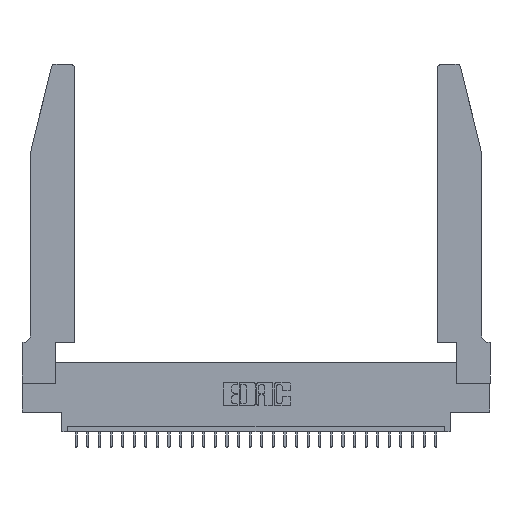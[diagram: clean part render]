
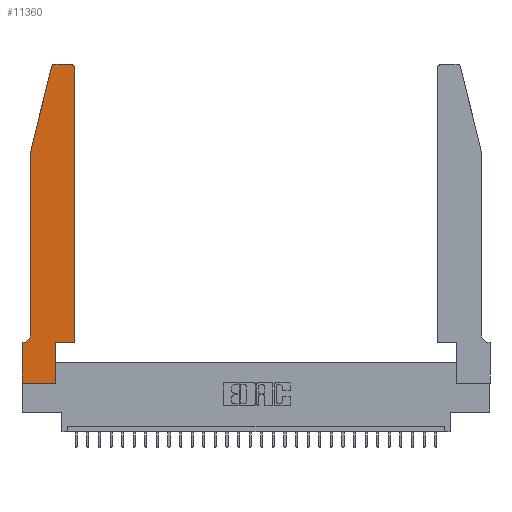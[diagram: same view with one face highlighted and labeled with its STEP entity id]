
A CAD part, top view. The second image highlights one B-rep face of the part: STEP entity #11360.
In plain terms, the highlighted planar face has unit normal (0, 0, 1).
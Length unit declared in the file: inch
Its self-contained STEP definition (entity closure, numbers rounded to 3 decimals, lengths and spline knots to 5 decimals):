
#20 = CARTESIAN_POINT ( 'NONE',  ( 0.4505, 0.35, 0.37 ) ) ;
#382 = VERTEX_POINT ( 'NONE', #9187 ) ;
#573 = CARTESIAN_POINT ( 'NONE',  ( 0.2865, 0.35, 0.37 ) ) ;
#619 = CARTESIAN_POINT ( 'NONE',  ( 0.0755, 0.35, 0.37 ) ) ;
#842 = DIRECTION ( 'NONE',  ( -1., 0., 0. ) ) ;
#876 = ORIENTED_EDGE ( 'NONE', *, *, #18215, .T. ) ;
#1455 = DIRECTION ( 'NONE',  ( 0., -1., 0. ) ) ;
#1483 = VERTEX_POINT ( 'NONE', #17665 ) ;
#1603 = CARTESIAN_POINT ( 'NONE',  ( 0., 0., 0.37 ) ) ;
#1995 = VECTOR ( 'NONE', #14037, 39.37008 ) ;
#2484 = VERTEX_POINT ( 'NONE', #15204 ) ;
#2907 = PLANE ( 'NONE',  #17124 ) ;
#3189 = CARTESIAN_POINT ( 'NONE',  ( 0., 0.35, 0.37 ) ) ;
#3378 = EDGE_CURVE ( 'NONE', #382, #1483, #17438, .T. ) ;
#3645 = DIRECTION ( 'NONE',  ( 0., -1., 0. ) ) ;
#4342 = DIRECTION ( 'NONE',  ( 1., 0., 0. ) ) ;
#4377 = CARTESIAN_POINT ( 'NONE',  ( 0.2865, 0.35, 0.37 ) ) ;
#4660 = LINE ( 'NONE', #9275, #1995 ) ;
#4884 = ORIENTED_EDGE ( 'NONE', *, *, #12506, .T. ) ;
#5061 = DIRECTION ( 'NONE',  ( 1., 0., 0. ) ) ;
#5172 = VECTOR ( 'NONE', #842, 39.37008 ) ;
#5564 = ORIENTED_EDGE ( 'NONE', *, *, #29871, .T. ) ;
#5565 = CIRCLE ( 'NONE', #13930, 0.07 ) ;
#5579 = EDGE_CURVE ( 'NONE', #24609, #23408, #24200, .T. ) ;
#5782 = ORIENTED_EDGE ( 'NONE', *, *, #13858, .T. ) ;
#5947 = AXIS2_PLACEMENT_3D ( 'NONE', #16611, #11855, #9076 ) ;
#6278 = CARTESIAN_POINT ( 'NONE',  ( 0.4205, 2.75, 0.37 ) ) ;
#6352 = EDGE_CURVE ( 'NONE', #14326, #21871, #22764, .T. ) ;
#7687 = CARTESIAN_POINT ( 'NONE',  ( 0.4505, 0.35, 0.37 ) ) ;
#7691 = DIRECTION ( 'NONE',  ( 0., 0., -1. ) ) ;
#8004 = VECTOR ( 'NONE', #28837, 39.37008 ) ;
#8402 = CIRCLE ( 'NONE', #5947, 0.03 ) ;
#9076 = DIRECTION ( 'NONE',  ( 1., 0., 0. ) ) ;
#9187 = CARTESIAN_POINT ( 'NONE',  ( 0.25487, 2.72718, 0.37 ) ) ;
#9194 = VECTOR ( 'NONE', #10585, 39.37008 ) ;
#9275 = CARTESIAN_POINT ( 'NONE',  ( 0., 0., 0.37 ) ) ;
#10516 = ORIENTED_EDGE ( 'NONE', *, *, #6352, .T. ) ;
#10585 = DIRECTION ( 'NONE',  ( -1., 0., 0. ) ) ;
#10731 = CARTESIAN_POINT ( 'NONE',  ( 0.0755, 2., 0.37 ) ) ;
#10820 = CARTESIAN_POINT ( 'NONE',  ( 0.0755, 0.42, 0.37 ) ) ;
#10958 = CARTESIAN_POINT ( 'NONE',  ( 0.0055, 0.35, 0.37 ) ) ;
#11006 = ORIENTED_EDGE ( 'NONE', *, *, #14253, .T. ) ;
#11298 = DIRECTION ( 'NONE',  ( 0., 1., 0. ) ) ;
#11360 = ADVANCED_FACE ( 'NONE', ( #19342 ), #2907, .T. ) ;
#11855 = DIRECTION ( 'NONE',  ( 0., 0., 1. ) ) ;
#11997 = CARTESIAN_POINT ( 'NONE',  ( 0., 0., 0.37 ) ) ;
#12376 = ORIENTED_EDGE ( 'NONE', *, *, #24326, .T. ) ;
#12506 = EDGE_CURVE ( 'NONE', #15424, #27310, #26975, .T. ) ;
#12516 = ORIENTED_EDGE ( 'NONE', *, *, #5579, .T. ) ;
#12882 = LINE ( 'NONE', #10731, #24291 ) ;
#13235 = EDGE_LOOP ( 'NONE', ( #12516, #12376, #16397, #876, #23222, #5564, #4884, #5782, #14923, #13460, #10516, #11006 ) ) ;
#13460 = ORIENTED_EDGE ( 'NONE', *, *, #30182, .T. ) ;
#13858 = EDGE_CURVE ( 'NONE', #27310, #2484, #4660, .T. ) ;
#13930 = AXIS2_PLACEMENT_3D ( 'NONE', #19076, #7691, #26302 ) ;
#13954 = DIRECTION ( 'NONE',  ( 1., 0., 0. ) ) ;
#14017 = VECTOR ( 'NONE', #26150, 39.37008 ) ;
#14037 = DIRECTION ( 'NONE',  ( 1., 0., 0. ) ) ;
#14253 = EDGE_CURVE ( 'NONE', #21871, #24609, #8402, .T. ) ;
#14326 = VERTEX_POINT ( 'NONE', #20 ) ;
#14923 = ORIENTED_EDGE ( 'NONE', *, *, #22488, .T. ) ;
#15204 = CARTESIAN_POINT ( 'NONE',  ( 0.2865, 0., 0.37 ) ) ;
#15424 = VERTEX_POINT ( 'NONE', #19080 ) ;
#16073 = EDGE_CURVE ( 'NONE', #28060, #28094, #5565, .T. ) ;
#16397 = ORIENTED_EDGE ( 'NONE', *, *, #3378, .T. ) ;
#16611 = CARTESIAN_POINT ( 'NONE',  ( 0.4205, 2.72, 0.37 ) ) ;
#17124 = AXIS2_PLACEMENT_3D ( 'NONE', #3189, #24114, #5061 ) ;
#17438 = LINE ( 'NONE', #26987, #8004 ) ;
#17665 = CARTESIAN_POINT ( 'NONE',  ( 0.0755, 2., 0.37 ) ) ;
#18136 = VECTOR ( 'NONE', #1455, 39.37008 ) ;
#18215 = EDGE_CURVE ( 'NONE', #1483, #28060, #12882, .T. ) ;
#19076 = CARTESIAN_POINT ( 'NONE',  ( 0.0055, 0.42, 0.37 ) ) ;
#19080 = CARTESIAN_POINT ( 'NONE',  ( 0., 0.35, 0.37 ) ) ;
#19335 = CARTESIAN_POINT ( 'NONE',  ( 0.4505, 2.72, 0.37 ) ) ;
#19342 = FACE_OUTER_BOUND ( 'NONE', #13235, .T. ) ;
#20000 = VECTOR ( 'NONE', #11298, 39.37008 ) ;
#21805 = LINE ( 'NONE', #619, #9194 ) ;
#21871 = VERTEX_POINT ( 'NONE', #19335 ) ;
#22254 = VERTEX_POINT ( 'NONE', #573 ) ;
#22488 = EDGE_CURVE ( 'NONE', #2484, #22254, #23433, .T. ) ;
#22764 = LINE ( 'NONE', #7687, #14017 ) ;
#23007 = CIRCLE ( 'NONE', #26947, 0.03 ) ;
#23222 = ORIENTED_EDGE ( 'NONE', *, *, #16073, .T. ) ;
#23325 = CARTESIAN_POINT ( 'NONE',  ( 0.4505, 0.35, 0.37 ) ) ;
#23408 = VERTEX_POINT ( 'NONE', #25943 ) ;
#23433 = LINE ( 'NONE', #4377, #20000 ) ;
#23698 = CARTESIAN_POINT ( 'NONE',  ( 0.284, 2.72, 0.37 ) ) ;
#24114 = DIRECTION ( 'NONE',  ( 0., 0., 1. ) ) ;
#24200 = LINE ( 'NONE', #24346, #5172 ) ;
#24291 = VECTOR ( 'NONE', #3645, 39.37008 ) ;
#24326 = EDGE_CURVE ( 'NONE', #23408, #382, #23007, .T. ) ;
#24346 = CARTESIAN_POINT ( 'NONE',  ( 0.2605, 2.75, 0.37 ) ) ;
#24609 = VERTEX_POINT ( 'NONE', #6278 ) ;
#24882 = VECTOR ( 'NONE', #13954, 39.37008 ) ;
#25943 = CARTESIAN_POINT ( 'NONE',  ( 0.284, 2.75, 0.37 ) ) ;
#25957 = LINE ( 'NONE', #23325, #24882 ) ;
#26022 = DIRECTION ( 'NONE',  ( 0., 0., 1. ) ) ;
#26150 = DIRECTION ( 'NONE',  ( 0., 1., 0. ) ) ;
#26302 = DIRECTION ( 'NONE',  ( -1., 0., 0. ) ) ;
#26947 = AXIS2_PLACEMENT_3D ( 'NONE', #23698, #26022, #4342 ) ;
#26975 = LINE ( 'NONE', #1603, #18136 ) ;
#26987 = CARTESIAN_POINT ( 'NONE',  ( 0.0755, 2., 0.37 ) ) ;
#27310 = VERTEX_POINT ( 'NONE', #11997 ) ;
#28060 = VERTEX_POINT ( 'NONE', #10820 ) ;
#28094 = VERTEX_POINT ( 'NONE', #10958 ) ;
#28837 = DIRECTION ( 'NONE',  ( -0.239, -0.971, 0. ) ) ;
#29871 = EDGE_CURVE ( 'NONE', #28094, #15424, #21805, .T. ) ;
#30182 = EDGE_CURVE ( 'NONE', #22254, #14326, #25957, .T. ) ;
